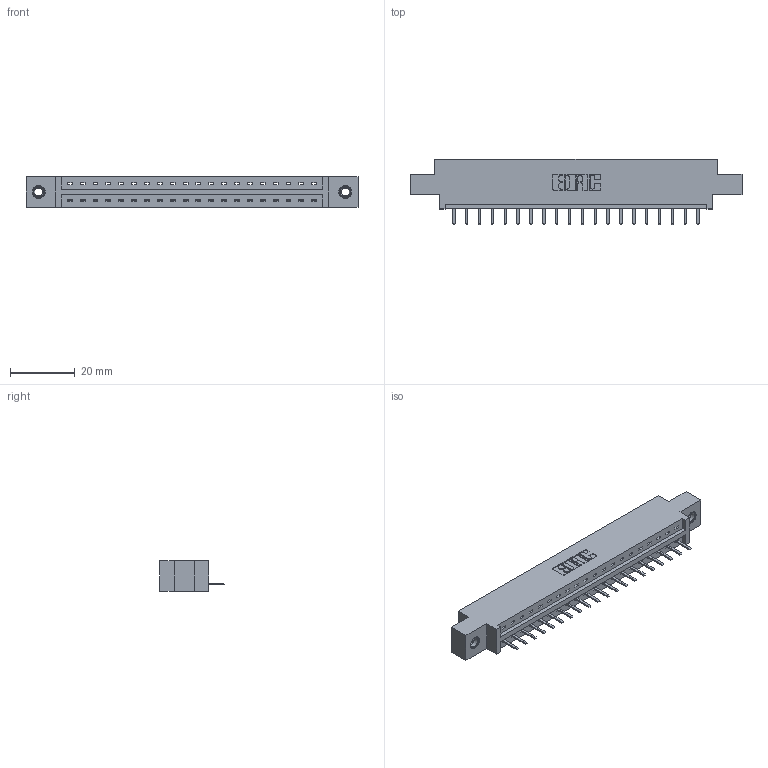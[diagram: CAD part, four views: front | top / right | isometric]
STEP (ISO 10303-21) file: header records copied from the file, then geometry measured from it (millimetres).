
FILE_DESCRIPTION (( 'STEP AP203' ), '1' );
FILE_NAME ('337-020-520-607.STEP', '2018-08-05T08:14:53', ( '' ), ( '' ), 'SwSTEP 2.0', 'SolidWorks 2016', '' );
FILE_SCHEMA (( 'CONFIG_CONTROL_DESIGN' ));
Length unit declared in the file: inch
Products named in the file (4): 337-020-520-607; 337 Part_0.170 Offset - 0.156 Dia-TI; 345-292-001_345-293-120; 345-250-001_345-250-005-103
Assembly tree (23 placements, depth 2):
  337-020-520-607
    337 Part_0.170 Offset - 0.156 Dia-TI
    345-292-001_345-293-120  x20
    345-250-001_345-250-005-103  x2
Bounding box: 102.26 x 20.02 x 9.4 mm (x, y, z)
Volume: 10164.4 mm3; surface area: 10311.7 mm2
Topology: 23 solids, 23 shells, 1498 faces, 4379 edges, 2858 vertices
Faces by surface type: plane 1066, cylinder 416, cone 12, torus 4
Entity records: 19144 total; most frequent: CARTESIAN_POINT 3325, ORIENTED_EDGE 3262, DIRECTION 2865, EDGE_CURVE 1631, VECTOR 1479, LINE 1479, VERTEX_POINT 1080, AXIS2_PLACEMENT_3D 693
